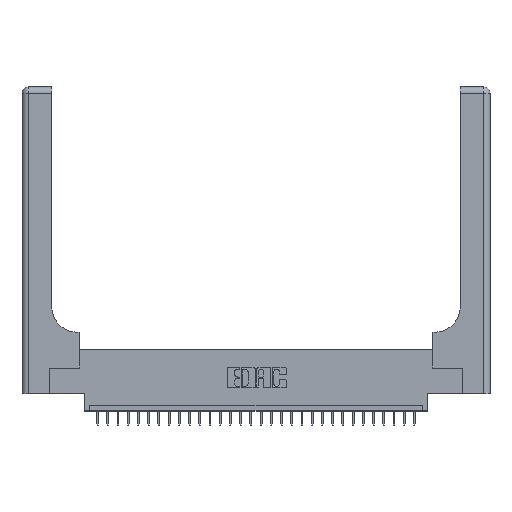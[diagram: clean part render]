
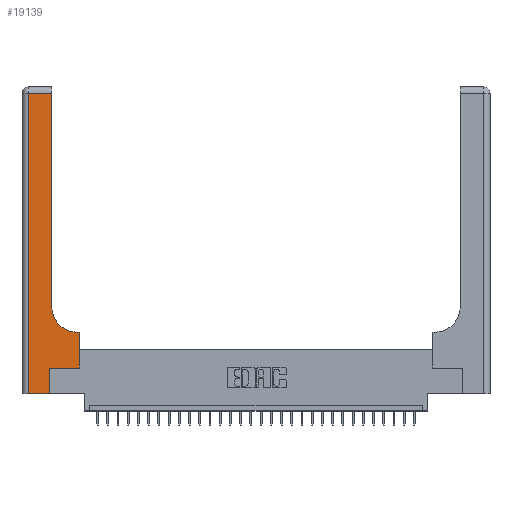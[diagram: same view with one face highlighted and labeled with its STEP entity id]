
A CAD part, top view. The second image highlights one B-rep face of the part: STEP entity #19139.
In plain terms, the highlighted planar face has unit normal (0, 0, 1).
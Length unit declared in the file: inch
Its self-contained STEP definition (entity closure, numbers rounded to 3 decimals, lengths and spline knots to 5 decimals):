
#1708 = LINE ( 'NONE', #11243, #18400 ) ;
#1848 = LINE ( 'NONE', #21252, #30344 ) ;
#2127 = EDGE_CURVE ( 'NONE', #12194, #25088, #1848, .T. ) ;
#2294 = ORIENTED_EDGE ( 'NONE', *, *, #20366, .T. ) ;
#2508 = CARTESIAN_POINT ( 'NONE',  ( 0.06, 0., 0.37 ) ) ;
#3437 = VECTOR ( 'NONE', #15383, 39.37008 ) ;
#3662 = CARTESIAN_POINT ( 'NONE',  ( 0.5415, 0.85, 0.37 ) ) ;
#3814 = VECTOR ( 'NONE', #15728, 39.37008 ) ;
#4386 = AXIS2_PLACEMENT_3D ( 'NONE', #22668, #16112, #18139 ) ;
#4457 = ORIENTED_EDGE ( 'NONE', *, *, #7508, .T. ) ;
#5195 = CARTESIAN_POINT ( 'NONE',  ( 0.2915, 0.85, 0.37 ) ) ;
#5410 = DIRECTION ( 'NONE',  ( 0., 1., 0. ) ) ;
#5840 = CARTESIAN_POINT ( 'NONE',  ( 0.2915, 3., 0.37 ) ) ;
#6529 = DIRECTION ( 'NONE',  ( 1., 0., 0. ) ) ;
#7273 = VERTEX_POINT ( 'NONE', #26489 ) ;
#7508 = EDGE_CURVE ( 'NONE', #7610, #30531, #23966, .T. ) ;
#7527 = ORIENTED_EDGE ( 'NONE', *, *, #20563, .T. ) ;
#7610 = VERTEX_POINT ( 'NONE', #11941 ) ;
#8017 = CARTESIAN_POINT ( 'NONE',  ( 0.5415, 0.6, 0.37 ) ) ;
#8214 = DIRECTION ( 'NONE',  ( 0., 0., -1. ) ) ;
#8758 = PLANE ( 'NONE',  #4386 ) ;
#9239 = VERTEX_POINT ( 'NONE', #5195 ) ;
#10083 = VERTEX_POINT ( 'NONE', #28824 ) ;
#10476 = EDGE_CURVE ( 'NONE', #16559, #23525, #17766, .T. ) ;
#10878 = VECTOR ( 'NONE', #5410, 39.37008 ) ;
#11243 = CARTESIAN_POINT ( 'NONE',  ( 0., 0., 0.37 ) ) ;
#11747 = ORIENTED_EDGE ( 'NONE', *, *, #14664, .T. ) ;
#11941 = CARTESIAN_POINT ( 'NONE',  ( 0.269, 0., 0.37 ) ) ;
#11966 = LINE ( 'NONE', #21512, #10878 ) ;
#12194 = VERTEX_POINT ( 'NONE', #25504 ) ;
#13186 = LINE ( 'NONE', #5840, #3437 ) ;
#13250 = VECTOR ( 'NONE', #6529, 39.37008 ) ;
#14511 = EDGE_CURVE ( 'NONE', #7273, #16559, #11966, .T. ) ;
#14664 = EDGE_CURVE ( 'NONE', #23525, #9239, #21405, .T. ) ;
#15383 = DIRECTION ( 'NONE',  ( 0., 1., 0. ) ) ;
#15728 = DIRECTION ( 'NONE',  ( -1., 0., 0. ) ) ;
#16112 = DIRECTION ( 'NONE',  ( 0., 0., -1. ) ) ;
#16171 = VECTOR ( 'NONE', #16503, 39.37008 ) ;
#16503 = DIRECTION ( 'NONE',  ( 0., 1., 0. ) ) ;
#16559 = VERTEX_POINT ( 'NONE', #26092 ) ;
#17090 = ORIENTED_EDGE ( 'NONE', *, *, #29952, .T. ) ;
#17119 = ORIENTED_EDGE ( 'NONE', *, *, #2127, .T. ) ;
#17766 = LINE ( 'NONE', #17918, #3814 ) ;
#17918 = CARTESIAN_POINT ( 'NONE',  ( 0.2915, 0.6, 0.37 ) ) ;
#18139 = DIRECTION ( 'NONE',  ( -1., 0., 0. ) ) ;
#18252 = CARTESIAN_POINT ( 'NONE',  ( 0.269, 0.25, 0.37 ) ) ;
#18259 = EDGE_CURVE ( 'NONE', #25088, #7610, #1708, .T. ) ;
#18400 = VECTOR ( 'NONE', #20787, 39.37008 ) ;
#18527 = ORIENTED_EDGE ( 'NONE', *, *, #14511, .T. ) ;
#19110 = DIRECTION ( 'NONE',  ( -1., 0., 0. ) ) ;
#19139 = ADVANCED_FACE ( 'NONE', ( #25299 ), #8758, .F. ) ;
#19916 = VECTOR ( 'NONE', #19110, 39.37008 ) ;
#20084 = DIRECTION ( 'NONE',  ( 1., 0., 0. ) ) ;
#20366 = EDGE_CURVE ( 'NONE', #9239, #10083, #13186, .T. ) ;
#20563 = EDGE_CURVE ( 'NONE', #10083, #12194, #24400, .T. ) ;
#20787 = DIRECTION ( 'NONE',  ( 1., 0., 0. ) ) ;
#21252 = CARTESIAN_POINT ( 'NONE',  ( 0.06, 3., 0.37 ) ) ;
#21405 = CIRCLE ( 'NONE', #28332, 0.25 ) ;
#21512 = CARTESIAN_POINT ( 'NONE',  ( 0.5585, 0.25, 0.37 ) ) ;
#22107 = EDGE_LOOP ( 'NONE', ( #2294, #7527, #17119, #23556, #4457, #17090, #18527, #23980, #11747 ) ) ;
#22668 = CARTESIAN_POINT ( 'NONE',  ( 0., 3., 0.37 ) ) ;
#23525 = VERTEX_POINT ( 'NONE', #8017 ) ;
#23556 = ORIENTED_EDGE ( 'NONE', *, *, #18259, .T. ) ;
#23571 = DIRECTION ( 'NONE',  ( 0., -1., 0. ) ) ;
#23807 = CARTESIAN_POINT ( 'NONE',  ( 0.269, 0., 0.37 ) ) ;
#23966 = LINE ( 'NONE', #23807, #16171 ) ;
#23980 = ORIENTED_EDGE ( 'NONE', *, *, #10476, .T. ) ;
#24400 = LINE ( 'NONE', #26722, #19916 ) ;
#25088 = VERTEX_POINT ( 'NONE', #2508 ) ;
#25299 = FACE_OUTER_BOUND ( 'NONE', #22107, .T. ) ;
#25504 = CARTESIAN_POINT ( 'NONE',  ( 0.06, 2.94, 0.37 ) ) ;
#25712 = LINE ( 'NONE', #18252, #13250 ) ;
#26092 = CARTESIAN_POINT ( 'NONE',  ( 0.5585, 0.6, 0.37 ) ) ;
#26489 = CARTESIAN_POINT ( 'NONE',  ( 0.5585, 0.25, 0.37 ) ) ;
#26722 = CARTESIAN_POINT ( 'NONE',  ( 0., 2.94, 0.37 ) ) ;
#28332 = AXIS2_PLACEMENT_3D ( 'NONE', #3662, #8214, #20084 ) ;
#28824 = CARTESIAN_POINT ( 'NONE',  ( 0.2915, 2.94, 0.37 ) ) ;
#29271 = CARTESIAN_POINT ( 'NONE',  ( 0.269, 0.25, 0.37 ) ) ;
#29952 = EDGE_CURVE ( 'NONE', #30531, #7273, #25712, .T. ) ;
#30344 = VECTOR ( 'NONE', #23571, 39.37008 ) ;
#30531 = VERTEX_POINT ( 'NONE', #29271 ) ;
